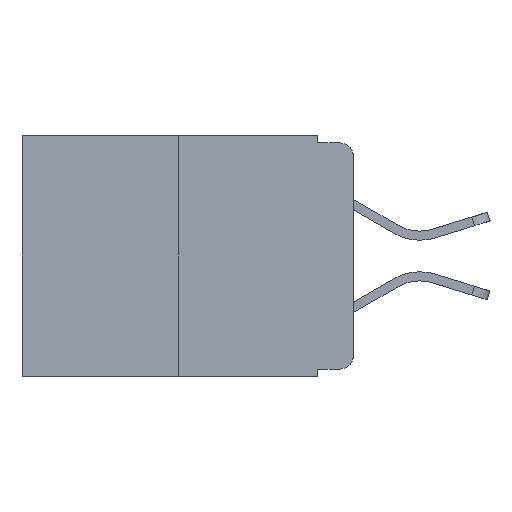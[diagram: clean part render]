
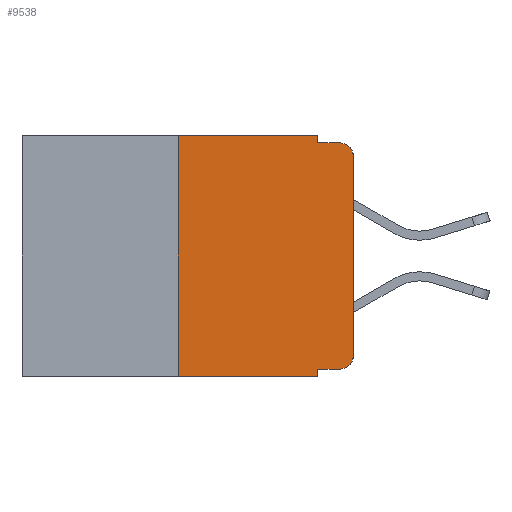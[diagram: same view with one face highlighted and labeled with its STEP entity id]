
A CAD part, left-side view. The second image highlights one B-rep face of the part: STEP entity #9538.
In plain terms, the highlighted planar face has unit normal (-1, 0, 0).
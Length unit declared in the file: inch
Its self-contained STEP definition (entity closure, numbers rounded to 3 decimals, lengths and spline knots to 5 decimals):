
#23 = ORIENTED_EDGE ( 'NONE', *, *, #625, .F. ) ;
#205 = DIRECTION ( 'NONE',  ( 0., -1., 0. ) ) ;
#415 = DIRECTION ( 'NONE',  ( 0., 0., -1. ) ) ;
#583 = CARTESIAN_POINT ( 'NONE',  ( 0., 0.02, -0.03 ) ) ;
#625 = EDGE_CURVE ( 'NONE', #6530, #2348, #11832, .T. ) ;
#1141 = ORIENTED_EDGE ( 'NONE', *, *, #9447, .F. ) ;
#1264 = EDGE_CURVE ( 'NONE', #19594, #9729, #18880, .T. ) ;
#1379 = VERTEX_POINT ( 'NONE', #21896 ) ;
#1443 = FACE_OUTER_BOUND ( 'NONE', #10605, .T. ) ;
#1865 = CARTESIAN_POINT ( 'NONE',  ( 0., 0.051, 0. ) ) ;
#1888 = CARTESIAN_POINT ( 'NONE',  ( 0., 0.02, -0.333 ) ) ;
#2348 = VERTEX_POINT ( 'NONE', #19351 ) ;
#2440 = DIRECTION ( 'NONE',  ( 0., 0., -1. ) ) ;
#2487 = CARTESIAN_POINT ( 'NONE',  ( 0., 0.051, 0. ) ) ;
#2637 = AXIS2_PLACEMENT_3D ( 'NONE', #583, #13155, #2440 ) ;
#2649 = VERTEX_POINT ( 'NONE', #2487 ) ;
#2885 = ORIENTED_EDGE ( 'NONE', *, *, #1264, .T. ) ;
#3347 = VERTEX_POINT ( 'NONE', #16815 ) ;
#3640 = VERTEX_POINT ( 'NONE', #19818 ) ;
#3923 = DIRECTION ( 'NONE',  ( 0., 0., 1. ) ) ;
#4134 = CARTESIAN_POINT ( 'NONE',  ( 0., 0.051, -0.01 ) ) ;
#4204 = PLANE ( 'NONE',  #17205 ) ;
#4313 = DIRECTION ( 'NONE',  ( 0., 0., 1. ) ) ;
#4712 = EDGE_CURVE ( 'NONE', #19070, #19594, #5994, .T. ) ;
#4807 = LINE ( 'NONE', #21446, #22384 ) ;
#5015 = ORIENTED_EDGE ( 'NONE', *, *, #16145, .F. ) ;
#5556 = VERTEX_POINT ( 'NONE', #4134 ) ;
#5726 = ORIENTED_EDGE ( 'NONE', *, *, #16901, .T. ) ;
#5994 = CIRCLE ( 'NONE', #20627, 0.02 ) ;
#6451 = VECTOR ( 'NONE', #20492, 39.37008 ) ;
#6530 = VERTEX_POINT ( 'NONE', #20698 ) ;
#6824 = DIRECTION ( 'NONE',  ( -1., 0., 0. ) ) ;
#6846 = VECTOR ( 'NONE', #14586, 39.37008 ) ;
#7182 = CARTESIAN_POINT ( 'NONE',  ( 0., 0., -0.313 ) ) ;
#7808 = CARTESIAN_POINT ( 'NONE',  ( 0., 0.473, 0. ) ) ;
#9447 = EDGE_CURVE ( 'NONE', #5556, #3347, #11565, .T. ) ;
#9538 = ADVANCED_FACE ( 'NONE', ( #1443 ), #4204, .F. ) ;
#9673 = CARTESIAN_POINT ( 'NONE',  ( 0., 0.473, 0. ) ) ;
#9729 = VERTEX_POINT ( 'NONE', #15212 ) ;
#9921 = CARTESIAN_POINT ( 'NONE',  ( 0., 0.051, -0.333 ) ) ;
#9993 = CARTESIAN_POINT ( 'NONE',  ( 0., 0.051, 0. ) ) ;
#10514 = ORIENTED_EDGE ( 'NONE', *, *, #11357, .T. ) ;
#10605 = EDGE_LOOP ( 'NONE', ( #2885, #20705, #1141, #18564, #11101, #5015, #10514, #23, #5726, #19567 ) ) ;
#11101 = ORIENTED_EDGE ( 'NONE', *, *, #15570, .F. ) ;
#11192 = LINE ( 'NONE', #9993, #6451 ) ;
#11357 = EDGE_CURVE ( 'NONE', #1379, #2348, #4807, .T. ) ;
#11371 = DIRECTION ( 'NONE',  ( 0., 0., -1. ) ) ;
#11514 = VECTOR ( 'NONE', #11683, 39.37008 ) ;
#11565 = LINE ( 'NONE', #21494, #6846 ) ;
#11683 = DIRECTION ( 'NONE',  ( 0., -1., 0. ) ) ;
#11832 = LINE ( 'NONE', #1865, #21622 ) ;
#12148 = VECTOR ( 'NONE', #20108, 39.37008 ) ;
#12245 = EDGE_CURVE ( 'NONE', #2649, #5556, #11192, .T. ) ;
#13155 = DIRECTION ( 'NONE',  ( -1., 0., 0. ) ) ;
#14586 = DIRECTION ( 'NONE',  ( 0., -1., 0. ) ) ;
#14626 = CARTESIAN_POINT ( 'NONE',  ( 0., 0., 0. ) ) ;
#14928 = CARTESIAN_POINT ( 'NONE',  ( 0., 0.25, 0. ) ) ;
#15212 = CARTESIAN_POINT ( 'NONE',  ( 0., 0., -0.03 ) ) ;
#15570 = EDGE_CURVE ( 'NONE', #3640, #2649, #21920, .T. ) ;
#16145 = EDGE_CURVE ( 'NONE', #1379, #3640, #21616, .T. ) ;
#16760 = EDGE_CURVE ( 'NONE', #9729, #3347, #18873, .T. ) ;
#16815 = CARTESIAN_POINT ( 'NONE',  ( 0., 0.02, -0.01 ) ) ;
#16901 = EDGE_CURVE ( 'NONE', #6530, #19070, #20772, .T. ) ;
#17003 = VECTOR ( 'NONE', #4313, 39.37008 ) ;
#17205 = AXIS2_PLACEMENT_3D ( 'NONE', #7808, #21781, #11371 ) ;
#17359 = CARTESIAN_POINT ( 'NONE',  ( 0., 0.02, -0.313 ) ) ;
#18086 = VECTOR ( 'NONE', #3923, 39.37008 ) ;
#18564 = ORIENTED_EDGE ( 'NONE', *, *, #12245, .F. ) ;
#18873 = CIRCLE ( 'NONE', #2637, 0.02 ) ;
#18880 = LINE ( 'NONE', #14626, #18086 ) ;
#19070 = VERTEX_POINT ( 'NONE', #1888 ) ;
#19094 = DIRECTION ( 'NONE',  ( 0., 0., -1. ) ) ;
#19351 = CARTESIAN_POINT ( 'NONE',  ( 0., 0.051, -0.343 ) ) ;
#19567 = ORIENTED_EDGE ( 'NONE', *, *, #4712, .T. ) ;
#19594 = VERTEX_POINT ( 'NONE', #7182 ) ;
#19818 = CARTESIAN_POINT ( 'NONE',  ( 0., 0.25, 0. ) ) ;
#20108 = DIRECTION ( 'NONE',  ( 0., -1., 0. ) ) ;
#20492 = DIRECTION ( 'NONE',  ( 0., 0., -1. ) ) ;
#20627 = AXIS2_PLACEMENT_3D ( 'NONE', #17359, #6824, #19094 ) ;
#20698 = CARTESIAN_POINT ( 'NONE',  ( 0., 0.051, -0.333 ) ) ;
#20705 = ORIENTED_EDGE ( 'NONE', *, *, #16760, .T. ) ;
#20772 = LINE ( 'NONE', #9921, #11514 ) ;
#21446 = CARTESIAN_POINT ( 'NONE',  ( 0., 0.473, -0.343 ) ) ;
#21494 = CARTESIAN_POINT ( 'NONE',  ( 0., 0.051, -0.01 ) ) ;
#21616 = LINE ( 'NONE', #14928, #17003 ) ;
#21622 = VECTOR ( 'NONE', #415, 39.37008 ) ;
#21781 = DIRECTION ( 'NONE',  ( 1., 0., 0. ) ) ;
#21896 = CARTESIAN_POINT ( 'NONE',  ( 0., 0.25, -0.343 ) ) ;
#21920 = LINE ( 'NONE', #9673, #12148 ) ;
#22384 = VECTOR ( 'NONE', #205, 39.37008 ) ;
